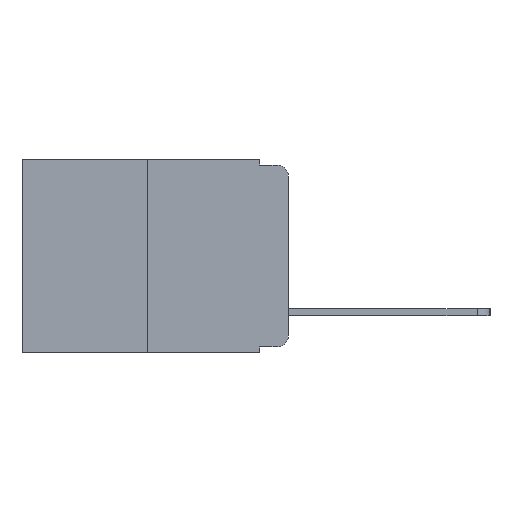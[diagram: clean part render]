
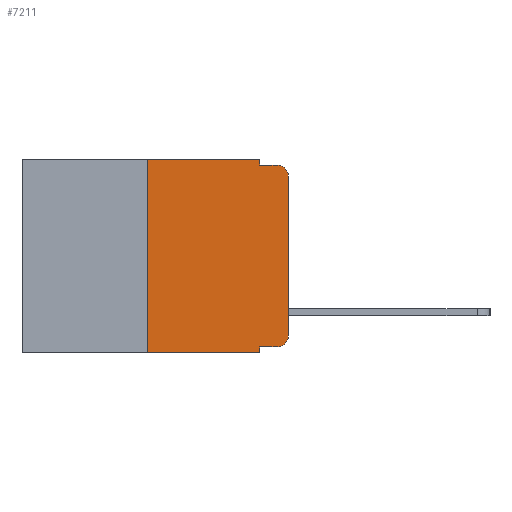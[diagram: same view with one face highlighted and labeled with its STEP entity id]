
A CAD part, left-side view. The second image highlights one B-rep face of the part: STEP entity #7211.
In plain terms, the highlighted planar face has unit normal (-1, 0, 0).
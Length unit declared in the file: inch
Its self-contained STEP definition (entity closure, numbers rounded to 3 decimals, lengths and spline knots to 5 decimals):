
#318 = DIRECTION ( 'NONE',  ( 0., 0., 1. ) ) ;
#428 = EDGE_CURVE ( 'NONE', #6236, #9629, #7967, .T. ) ;
#578 = VECTOR ( 'NONE', #1912, 39.37008 ) ;
#646 = VERTEX_POINT ( 'NONE', #8603 ) ;
#878 = ORIENTED_EDGE ( 'NONE', *, *, #8583, .T. ) ;
#1114 = CARTESIAN_POINT ( 'NONE',  ( 0., 0.02, -0.313 ) ) ;
#1294 = VECTOR ( 'NONE', #3083, 39.37008 ) ;
#1337 = EDGE_CURVE ( 'NONE', #4022, #9629, #2094, .T. ) ;
#1612 = VECTOR ( 'NONE', #4172, 39.37008 ) ;
#1697 = ORIENTED_EDGE ( 'NONE', *, *, #12589, .F. ) ;
#1896 = VERTEX_POINT ( 'NONE', #11547 ) ;
#1912 = DIRECTION ( 'NONE',  ( 0., -1., 0. ) ) ;
#2094 = LINE ( 'NONE', #4793, #12163 ) ;
#2098 = DIRECTION ( 'NONE',  ( 0., 0., 1. ) ) ;
#2125 = DIRECTION ( 'NONE',  ( 0., 0., -1. ) ) ;
#2128 = DIRECTION ( 'NONE',  ( 1., 0., 0. ) ) ;
#2377 = VECTOR ( 'NONE', #11200, 39.37008 ) ;
#2762 = VECTOR ( 'NONE', #10596, 39.37008 ) ;
#3083 = DIRECTION ( 'NONE',  ( 0., 0., -1. ) ) ;
#3161 = EDGE_CURVE ( 'NONE', #6921, #9895, #6234, .T. ) ;
#3167 = AXIS2_PLACEMENT_3D ( 'NONE', #1114, #8010, #2125 ) ;
#3202 = CARTESIAN_POINT ( 'NONE',  ( 0., 0.02, -0.333 ) ) ;
#3419 = CARTESIAN_POINT ( 'NONE',  ( 0., 0.051, -0.333 ) ) ;
#3576 = ORIENTED_EDGE ( 'NONE', *, *, #1337, .T. ) ;
#3587 = ORIENTED_EDGE ( 'NONE', *, *, #10219, .T. ) ;
#3736 = ORIENTED_EDGE ( 'NONE', *, *, #4555, .F. ) ;
#3926 = DIRECTION ( 'NONE',  ( 0., -1., 0. ) ) ;
#4022 = VERTEX_POINT ( 'NONE', #8342 ) ;
#4108 = PLANE ( 'NONE',  #11876 ) ;
#4172 = DIRECTION ( 'NONE',  ( 0., -1., 0. ) ) ;
#4271 = LINE ( 'NONE', #12761, #1294 ) ;
#4362 = AXIS2_PLACEMENT_3D ( 'NONE', #4784, #11579, #5784 ) ;
#4530 = LINE ( 'NONE', #7020, #11966 ) ;
#4555 = EDGE_CURVE ( 'NONE', #4022, #646, #4530, .T. ) ;
#4635 = VERTEX_POINT ( 'NONE', #3202 ) ;
#4643 = ORIENTED_EDGE ( 'NONE', *, *, #3161, .F. ) ;
#4784 = CARTESIAN_POINT ( 'NONE',  ( 0., 0.02, -0.03 ) ) ;
#4793 = CARTESIAN_POINT ( 'NONE',  ( 0., 0.473, -0.343 ) ) ;
#5111 = CARTESIAN_POINT ( 'NONE',  ( 0., 0.051, -0.343 ) ) ;
#5265 = ORIENTED_EDGE ( 'NONE', *, *, #5637, .T. ) ;
#5497 = EDGE_CURVE ( 'NONE', #9229, #12384, #5731, .T. ) ;
#5637 = EDGE_CURVE ( 'NONE', #4635, #9229, #8787, .T. ) ;
#5731 = LINE ( 'NONE', #8270, #8329 ) ;
#5784 = DIRECTION ( 'NONE',  ( 0., 0., -1. ) ) ;
#6234 = LINE ( 'NONE', #7846, #578 ) ;
#6236 = VERTEX_POINT ( 'NONE', #3419 ) ;
#6408 = CARTESIAN_POINT ( 'NONE',  ( 0., 0.02, -0.01 ) ) ;
#6506 = ORIENTED_EDGE ( 'NONE', *, *, #5497, .T. ) ;
#6542 = CARTESIAN_POINT ( 'NONE',  ( 0., 0.051, -0.01 ) ) ;
#6589 = CIRCLE ( 'NONE', #4362, 0.02 ) ;
#6921 = VERTEX_POINT ( 'NONE', #6542 ) ;
#7020 = CARTESIAN_POINT ( 'NONE',  ( 0., 0.25, 0. ) ) ;
#7211 = ADVANCED_FACE ( 'NONE', ( #9208 ), #4108, .F. ) ;
#7601 = LINE ( 'NONE', #10229, #2377 ) ;
#7672 = CARTESIAN_POINT ( 'NONE',  ( 0., 0.051, 0. ) ) ;
#7846 = CARTESIAN_POINT ( 'NONE',  ( 0., 0.051, -0.01 ) ) ;
#7967 = LINE ( 'NONE', #7672, #2762 ) ;
#8010 = DIRECTION ( 'NONE',  ( -1., 0., 0. ) ) ;
#8038 = CARTESIAN_POINT ( 'NONE',  ( 0., 0.051, -0.333 ) ) ;
#8051 = CARTESIAN_POINT ( 'NONE',  ( 0., 0., -0.03 ) ) ;
#8270 = CARTESIAN_POINT ( 'NONE',  ( 0., 0., 0. ) ) ;
#8329 = VECTOR ( 'NONE', #318, 39.37008 ) ;
#8342 = CARTESIAN_POINT ( 'NONE',  ( 0., 0.25, -0.343 ) ) ;
#8499 = CARTESIAN_POINT ( 'NONE',  ( 0., 0., -0.313 ) ) ;
#8583 = EDGE_CURVE ( 'NONE', #6236, #4635, #9455, .T. ) ;
#8603 = CARTESIAN_POINT ( 'NONE',  ( 0., 0.25, 0. ) ) ;
#8787 = CIRCLE ( 'NONE', #3167, 0.02 ) ;
#9004 = DIRECTION ( 'NONE',  ( 0., 0., -1. ) ) ;
#9208 = FACE_OUTER_BOUND ( 'NONE', #10673, .T. ) ;
#9229 = VERTEX_POINT ( 'NONE', #8499 ) ;
#9455 = LINE ( 'NONE', #8038, #1612 ) ;
#9522 = ORIENTED_EDGE ( 'NONE', *, *, #11132, .F. ) ;
#9629 = VERTEX_POINT ( 'NONE', #5111 ) ;
#9895 = VERTEX_POINT ( 'NONE', #6408 ) ;
#10219 = EDGE_CURVE ( 'NONE', #12384, #9895, #6589, .T. ) ;
#10229 = CARTESIAN_POINT ( 'NONE',  ( 0., 0.473, 0. ) ) ;
#10596 = DIRECTION ( 'NONE',  ( 0., 0., -1. ) ) ;
#10673 = EDGE_LOOP ( 'NONE', ( #6506, #3587, #4643, #9522, #1697, #3736, #3576, #11091, #878, #5265 ) ) ;
#11091 = ORIENTED_EDGE ( 'NONE', *, *, #428, .F. ) ;
#11132 = EDGE_CURVE ( 'NONE', #1896, #6921, #4271, .T. ) ;
#11200 = DIRECTION ( 'NONE',  ( 0., -1., 0. ) ) ;
#11547 = CARTESIAN_POINT ( 'NONE',  ( 0., 0.051, 0. ) ) ;
#11579 = DIRECTION ( 'NONE',  ( -1., 0., 0. ) ) ;
#11849 = CARTESIAN_POINT ( 'NONE',  ( 0., 0.473, 0. ) ) ;
#11876 = AXIS2_PLACEMENT_3D ( 'NONE', #11849, #2128, #9004 ) ;
#11966 = VECTOR ( 'NONE', #2098, 39.37008 ) ;
#12163 = VECTOR ( 'NONE', #3926, 39.37008 ) ;
#12384 = VERTEX_POINT ( 'NONE', #8051 ) ;
#12589 = EDGE_CURVE ( 'NONE', #646, #1896, #7601, .T. ) ;
#12761 = CARTESIAN_POINT ( 'NONE',  ( 0., 0.051, 0. ) ) ;
